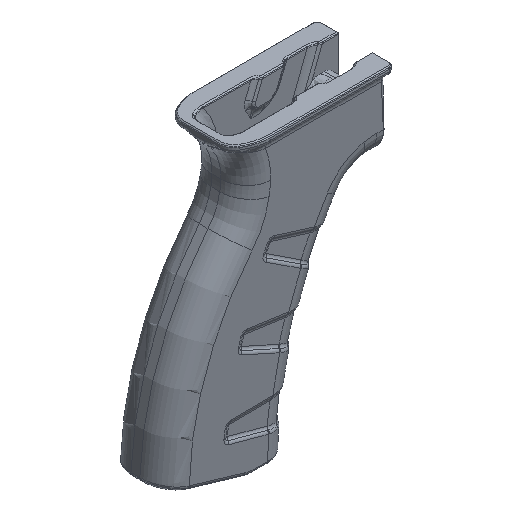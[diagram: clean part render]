
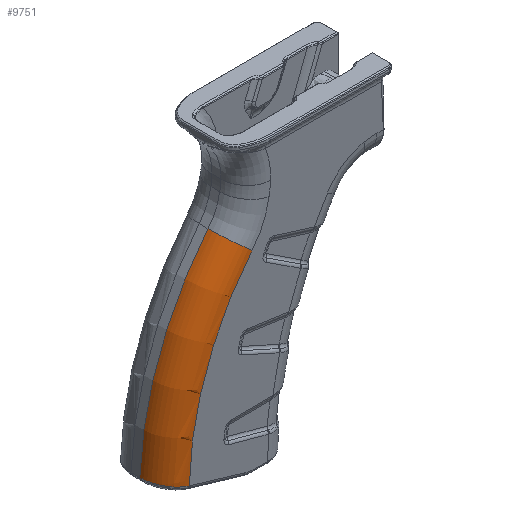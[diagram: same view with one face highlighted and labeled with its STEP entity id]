
A CAD part, isometric view. The second image highlights one B-rep face of the part: STEP entity #9751.
In plain terms, the highlighted toroidal (fillet/blend) face has major radius 101.565 mm and minor radius 9 mm.
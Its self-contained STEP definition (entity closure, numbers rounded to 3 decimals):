
#778=B_SPLINE_CURVE_WITH_KNOTS('',3,(#20359,#20360,#20361,#20362,#20363,
#20364),.UNSPECIFIED.,.F.,.F.,(4,1,1,4),(0.,0.55,0.916,
1.282),.UNSPECIFIED.);
#2166=FACE_OUTER_BOUND('',#2832,.T.);
#2832=EDGE_LOOP('',(#7864,#7865,#7866,#7867));
#3371=CIRCLE('',#10417,101.565);
#3443=CIRCLE('',#10516,110.565);
#3444=CIRCLE('',#10518,9.);
#4251=VERTEX_POINT('',#19140);
#4252=VERTEX_POINT('',#19142);
#4330=VERTEX_POINT('',#20348);
#4359=VERTEX_POINT('',#20937);
#5395=EDGE_CURVE('',#4251,#4252,#3371,.T.);
#5524=EDGE_CURVE('',#4252,#4330,#778,.T.);
#5581=EDGE_CURVE('',#4330,#4359,#3443,.T.);
#5583=EDGE_CURVE('',#4251,#4359,#3444,.T.);
#7864=ORIENTED_EDGE('',*,*,#5524,.F.);
#7865=ORIENTED_EDGE('',*,*,#5395,.F.);
#7866=ORIENTED_EDGE('',*,*,#5583,.T.);
#7867=ORIENTED_EDGE('',*,*,#5581,.F.);
#9358=TOROIDAL_SURFACE('',#10517,101.565,9.);
#9751=ADVANCED_FACE('',(#2166),#9358,.T.);
#10417=AXIS2_PLACEMENT_3D('',#19143,#11842,#11843);
#10516=AXIS2_PLACEMENT_3D('',#20938,#12077,#12078);
#10517=AXIS2_PLACEMENT_3D('',#20940,#12080,#12081);
#10518=AXIS2_PLACEMENT_3D('',#20941,#12082,#12083);
#11842=DIRECTION('center_axis',(0.,-1.,0.));
#11843=DIRECTION('ref_axis',(-0.79,0.,0.613));
#12077=DIRECTION('center_axis',(0.,1.,0.));
#12078=DIRECTION('ref_axis',(-0.79,0.,0.613));
#12080=DIRECTION('center_axis',(0.,-1.,0.));
#12081=DIRECTION('ref_axis',(0.,0.,1.));
#12082=DIRECTION('center_axis',(-0.631,0.,
-0.776));
#12083=DIRECTION('ref_axis',(0.,-1.,0.));
#19140=CARTESIAN_POINT('',(1.031,-10.6,-36.013));
#19142=CARTESIAN_POINT('',(-21.726,-10.6,-98.572));
#19143=CARTESIAN_POINT('Origin',(79.827,-10.6,-100.095));
#20348=CARTESIAN_POINT('',(-30.663,-1.6,-96.042));
#20359=CARTESIAN_POINT('Ctrl Pts',(-21.726,-10.6,-98.572));
#20360=CARTESIAN_POINT('Ctrl Pts',(-23.689,-10.6,
-98.007));
#20361=CARTESIAN_POINT('Ctrl Pts',(-26.969,-9.484,
-97.077));
#20362=CARTESIAN_POINT('Ctrl Pts',(-30.025,-5.717,
-96.22));
#20363=CARTESIAN_POINT('Ctrl Pts',(-30.663,-2.974,-96.042));
#20364=CARTESIAN_POINT('Ctrl Pts',(-30.663,-1.6,-96.042));
#20937=CARTESIAN_POINT('',(-5.951,-1.6,-30.334));
#20938=CARTESIAN_POINT('Origin',(79.827,-1.6,-100.095));
#20940=CARTESIAN_POINT('Origin',(79.827,-1.6,-100.095));
#20941=CARTESIAN_POINT('Origin',(1.031,-1.6,-36.013));
